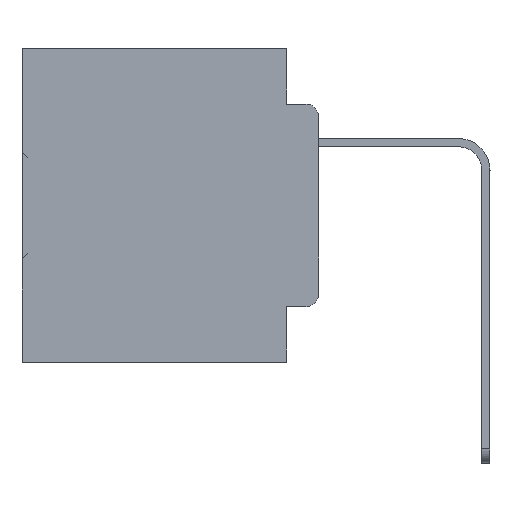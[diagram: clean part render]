
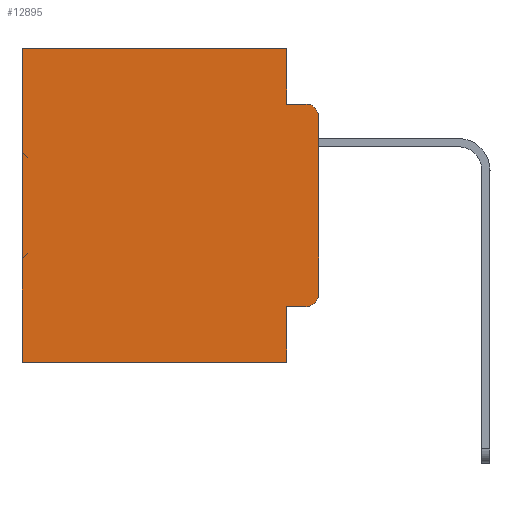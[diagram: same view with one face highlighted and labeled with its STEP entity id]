
A CAD part, left-side view. The second image highlights one B-rep face of the part: STEP entity #12895.
In plain terms, the highlighted planar face has unit normal (-1, 0, 0).
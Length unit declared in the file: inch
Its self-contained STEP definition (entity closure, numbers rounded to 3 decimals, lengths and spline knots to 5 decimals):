
#256 = VERTEX_POINT ( 'NONE', #10645 ) ;
#384 = CARTESIAN_POINT ( 'NONE',  ( 0.298, 0.051, 0. ) ) ;
#548 = ORIENTED_EDGE ( 'NONE', *, *, #28853, .F. ) ;
#817 = LINE ( 'NONE', #9323, #18033 ) ;
#838 = EDGE_CURVE ( 'NONE', #26555, #36521, #8449, .T. ) ;
#1564 = VECTOR ( 'NONE', #7928, 39.37008 ) ;
#1674 = LINE ( 'NONE', #36266, #26885 ) ;
#1677 = CARTESIAN_POINT ( 'NONE',  ( 0.298, 0., -0.3915 ) ) ;
#1808 = CARTESIAN_POINT ( 'NONE',  ( 0.298, 0.051, -0.5 ) ) ;
#1918 = CARTESIAN_POINT ( 'NONE',  ( 0.298, 0.02, -0.1085 ) ) ;
#2021 = VERTEX_POINT ( 'NONE', #19325 ) ;
#2097 = CARTESIAN_POINT ( 'NONE',  ( 0.298, 0.051, 0. ) ) ;
#2278 = CARTESIAN_POINT ( 'NONE',  ( 0.298, 0., 0. ) ) ;
#2475 = LINE ( 'NONE', #28900, #13055 ) ;
#3380 = FACE_OUTER_BOUND ( 'NONE', #15665, .T. ) ;
#4715 = EDGE_CURVE ( 'NONE', #256, #21641, #11686, .T. ) ;
#6100 = VERTEX_POINT ( 'NONE', #36340 ) ;
#6187 = ORIENTED_EDGE ( 'NONE', *, *, #7360, .T. ) ;
#7360 = EDGE_CURVE ( 'NONE', #21641, #36521, #29713, .T. ) ;
#7907 = CARTESIAN_POINT ( 'NONE',  ( 0.298, 0.051, -0.0885 ) ) ;
#7928 = DIRECTION ( 'NONE',  ( 0., -1., 0. ) ) ;
#8154 = ORIENTED_EDGE ( 'NONE', *, *, #33067, .F. ) ;
#8248 = AXIS2_PLACEMENT_3D ( 'NONE', #12632, #9900, #32419 ) ;
#8449 = LINE ( 'NONE', #27558, #21333 ) ;
#9323 = CARTESIAN_POINT ( 'NONE',  ( 0.298, 0.051, 0. ) ) ;
#9714 = DIRECTION ( 'NONE',  ( 0., 0., -1. ) ) ;
#9900 = DIRECTION ( 'NONE',  ( -1., 0., 0. ) ) ;
#10385 = DIRECTION ( 'NONE',  ( 0., 0., -1. ) ) ;
#10645 = CARTESIAN_POINT ( 'NONE',  ( 0.298, 0.051, -0.4115 ) ) ;
#11089 = VERTEX_POINT ( 'NONE', #7907 ) ;
#11130 = ORIENTED_EDGE ( 'NONE', *, *, #838, .F. ) ;
#11686 = LINE ( 'NONE', #22540, #1564 ) ;
#12064 = DIRECTION ( 'NONE',  ( 0., 0., -1. ) ) ;
#12630 = EDGE_CURVE ( 'NONE', #35475, #6100, #24658, .T. ) ;
#12632 = CARTESIAN_POINT ( 'NONE',  ( 0.298, 0.02, -0.3915 ) ) ;
#12895 = ADVANCED_FACE ( 'NONE', ( #3380 ), #24512, .F. ) ;
#13055 = VECTOR ( 'NONE', #31581, 39.37008 ) ;
#14211 = VERTEX_POINT ( 'NONE', #30951 ) ;
#14533 = VERTEX_POINT ( 'NONE', #1808 ) ;
#15081 = ORIENTED_EDGE ( 'NONE', *, *, #19396, .F. ) ;
#15470 = ORIENTED_EDGE ( 'NONE', *, *, #33308, .F. ) ;
#15665 = EDGE_LOOP ( 'NONE', ( #11130, #27307, #15470, #8154, #24164, #22621, #15081, #548, #36295, #6187 ) ) ;
#16200 = DIRECTION ( 'NONE',  ( 1., 0., 0. ) ) ;
#18033 = VECTOR ( 'NONE', #12064, 39.37008 ) ;
#19325 = CARTESIAN_POINT ( 'NONE',  ( 0.298, 0.02, -0.0885 ) ) ;
#19396 = EDGE_CURVE ( 'NONE', #14533, #14211, #2475, .T. ) ;
#20805 = EDGE_CURVE ( 'NONE', #6100, #14211, #25802, .T. ) ;
#21333 = VECTOR ( 'NONE', #9714, 39.37008 ) ;
#21641 = VERTEX_POINT ( 'NONE', #34542 ) ;
#22540 = CARTESIAN_POINT ( 'NONE',  ( 0.298, 0.051, -0.4115 ) ) ;
#22621 = ORIENTED_EDGE ( 'NONE', *, *, #20805, .T. ) ;
#24164 = ORIENTED_EDGE ( 'NONE', *, *, #12630, .T. ) ;
#24512 = PLANE ( 'NONE',  #29503 ) ;
#24658 = LINE ( 'NONE', #29006, #31282 ) ;
#25802 = LINE ( 'NONE', #36077, #31536 ) ;
#26555 = VERTEX_POINT ( 'NONE', #33980 ) ;
#26885 = VECTOR ( 'NONE', #33553, 39.37008 ) ;
#27307 = ORIENTED_EDGE ( 'NONE', *, *, #36442, .T. ) ;
#27558 = CARTESIAN_POINT ( 'NONE',  ( 0.298, 0., 0. ) ) ;
#27582 = DIRECTION ( 'NONE',  ( 0., 0., -1. ) ) ;
#27747 = DIRECTION ( 'NONE',  ( 0., 0., -1. ) ) ;
#28853 = EDGE_CURVE ( 'NONE', #256, #14533, #32586, .T. ) ;
#28900 = CARTESIAN_POINT ( 'NONE',  ( 0.298, 0., -0.5 ) ) ;
#29006 = CARTESIAN_POINT ( 'NONE',  ( 0.298, 0., 0. ) ) ;
#29370 = DIRECTION ( 'NONE',  ( 0., 1., 0. ) ) ;
#29503 = AXIS2_PLACEMENT_3D ( 'NONE', #2278, #16200, #27747 ) ;
#29713 = CIRCLE ( 'NONE', #8248, 0.02 ) ;
#30951 = CARTESIAN_POINT ( 'NONE',  ( 0.298, 0.473, -0.5 ) ) ;
#31282 = VECTOR ( 'NONE', #29370, 39.37008 ) ;
#31536 = VECTOR ( 'NONE', #10385, 39.37008 ) ;
#31581 = DIRECTION ( 'NONE',  ( 0., 1., 0. ) ) ;
#32419 = DIRECTION ( 'NONE',  ( 0., 0., -1. ) ) ;
#32586 = LINE ( 'NONE', #2097, #34756 ) ;
#33008 = AXIS2_PLACEMENT_3D ( 'NONE', #1918, #35979, #35619 ) ;
#33067 = EDGE_CURVE ( 'NONE', #35475, #11089, #817, .T. ) ;
#33294 = CIRCLE ( 'NONE', #33008, 0.02 ) ;
#33308 = EDGE_CURVE ( 'NONE', #11089, #2021, #1674, .T. ) ;
#33553 = DIRECTION ( 'NONE',  ( 0., -1., 0. ) ) ;
#33980 = CARTESIAN_POINT ( 'NONE',  ( 0.298, 0., -0.1085 ) ) ;
#34542 = CARTESIAN_POINT ( 'NONE',  ( 0.298, 0.02, -0.4115 ) ) ;
#34756 = VECTOR ( 'NONE', #27582, 39.37008 ) ;
#35475 = VERTEX_POINT ( 'NONE', #384 ) ;
#35619 = DIRECTION ( 'NONE',  ( 0., 0., -1. ) ) ;
#35979 = DIRECTION ( 'NONE',  ( -1., 0., 0. ) ) ;
#36077 = CARTESIAN_POINT ( 'NONE',  ( 0.298, 0.473, 0. ) ) ;
#36266 = CARTESIAN_POINT ( 'NONE',  ( 0.298, 0.051, -0.0885 ) ) ;
#36295 = ORIENTED_EDGE ( 'NONE', *, *, #4715, .T. ) ;
#36340 = CARTESIAN_POINT ( 'NONE',  ( 0.298, 0.473, 0. ) ) ;
#36442 = EDGE_CURVE ( 'NONE', #26555, #2021, #33294, .T. ) ;
#36521 = VERTEX_POINT ( 'NONE', #1677 ) ;
